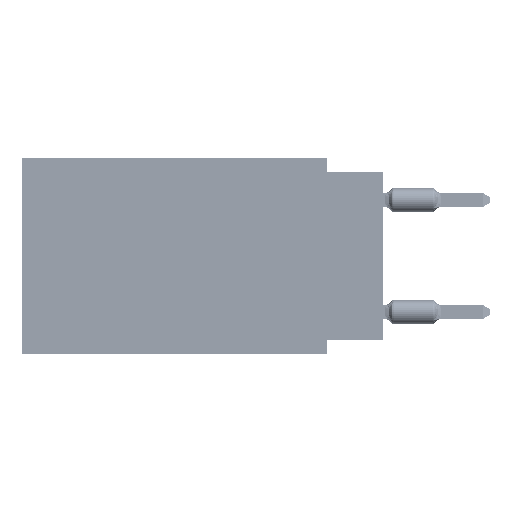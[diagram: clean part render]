
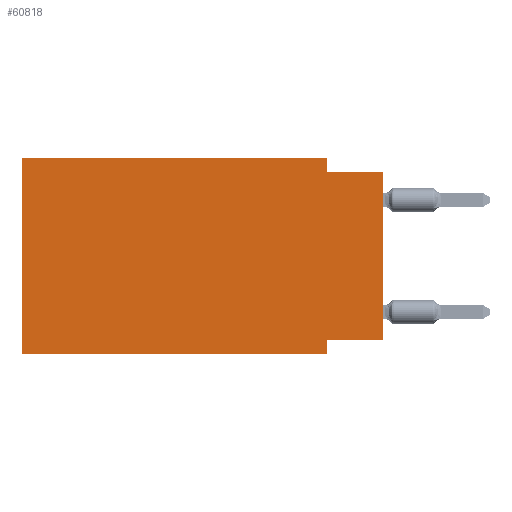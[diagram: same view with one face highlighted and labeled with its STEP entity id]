
A CAD part, left-side view. The second image highlights one B-rep face of the part: STEP entity #60818.
In plain terms, the highlighted planar face has unit normal (-1, 0, 0).
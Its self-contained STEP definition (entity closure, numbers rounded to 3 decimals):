
#2092 = DIRECTION ( 'NONE',  ( 0., -1., 0. ) ) ;
#2361 = LINE ( 'NONE', #91214, #15564 ) ;
#3045 = FACE_OUTER_BOUND ( 'NONE', #11937, .T. ) ;
#4152 = LINE ( 'NONE', #65462, #68832 ) ;
#7784 = CARTESIAN_POINT ( 'NONE',  ( 0., 0., -0.635 ) ) ;
#11937 = EDGE_LOOP ( 'NONE', ( #81461, #65099, #87087, #83864, #63018, #51238, #30250, #26063 ) ) ;
#12713 = AXIS2_PLACEMENT_3D ( 'NONE', #33919, #62898, #18721 ) ;
#15564 = VECTOR ( 'NONE', #53435, 1000. ) ;
#18721 = DIRECTION ( 'NONE',  ( 0., 0., -1. ) ) ;
#24284 = LINE ( 'NONE', #54211, #64107 ) ;
#25144 = CARTESIAN_POINT ( 'NONE',  ( 0., 0., -0.635 ) ) ;
#26063 = ORIENTED_EDGE ( 'NONE', *, *, #83132, .F. ) ;
#26356 = DIRECTION ( 'NONE',  ( 0., 0., 1. ) ) ;
#27761 = EDGE_CURVE ( 'NONE', #49866, #81852, #4152, .T. ) ;
#28850 = VERTEX_POINT ( 'NONE', #36926 ) ;
#29474 = CARTESIAN_POINT ( 'NONE',  ( 0., 2.54, -8.255 ) ) ;
#30038 = VECTOR ( 'NONE', #26356, 1000. ) ;
#30250 = ORIENTED_EDGE ( 'NONE', *, *, #27761, .F. ) ;
#30496 = VECTOR ( 'NONE', #78305, 1000. ) ;
#33228 = LINE ( 'NONE', #71983, #30038 ) ;
#33919 = CARTESIAN_POINT ( 'NONE',  ( 0., 16.383, 0. ) ) ;
#36542 = VERTEX_POINT ( 'NONE', #7784 ) ;
#36926 = CARTESIAN_POINT ( 'NONE',  ( 0., 16.383, 0. ) ) ;
#36971 = EDGE_CURVE ( 'NONE', #58294, #81852, #63474, .T. ) ;
#38929 = VECTOR ( 'NONE', #62022, 1000. ) ;
#42200 = CARTESIAN_POINT ( 'NONE',  ( 0., 16.383, 0. ) ) ;
#42896 = DIRECTION ( 'NONE',  ( 0., 0., -1. ) ) ;
#43327 = VERTEX_POINT ( 'NONE', #69070 ) ;
#44041 = VECTOR ( 'NONE', #2092, 1000. ) ;
#44327 = VERTEX_POINT ( 'NONE', #67769 ) ;
#47376 = LINE ( 'NONE', #62113, #30496 ) ;
#49866 = VERTEX_POINT ( 'NONE', #29474 ) ;
#50780 = EDGE_CURVE ( 'NONE', #59638, #36542, #69331, .T. ) ;
#51238 = ORIENTED_EDGE ( 'NONE', *, *, #36971, .T. ) ;
#51826 = EDGE_CURVE ( 'NONE', #44327, #36542, #33228, .T. ) ;
#53435 = DIRECTION ( 'NONE',  ( 0., 0., -1. ) ) ;
#54211 = CARTESIAN_POINT ( 'NONE',  ( 0., 0., -8.255 ) ) ;
#54282 = VECTOR ( 'NONE', #64767, 1000. ) ;
#58294 = VERTEX_POINT ( 'NONE', #81008 ) ;
#59638 = VERTEX_POINT ( 'NONE', #65173 ) ;
#60818 = ADVANCED_FACE ( 'NONE', ( #3045 ), #63864, .F. ) ;
#62022 = DIRECTION ( 'NONE',  ( 0., -1., 0. ) ) ;
#62113 = CARTESIAN_POINT ( 'NONE',  ( 0., 16.383, 0. ) ) ;
#62898 = DIRECTION ( 'NONE',  ( 1., 0., 0. ) ) ;
#63018 = ORIENTED_EDGE ( 'NONE', *, *, #68877, .F. ) ;
#63474 = LINE ( 'NONE', #86050, #38929 ) ;
#63864 = PLANE ( 'NONE',  #12713 ) ;
#64107 = VECTOR ( 'NONE', #84153, 1000. ) ;
#64767 = DIRECTION ( 'NONE',  ( 0., 0., 1. ) ) ;
#65099 = ORIENTED_EDGE ( 'NONE', *, *, #50780, .F. ) ;
#65148 = EDGE_CURVE ( 'NONE', #28850, #43327, #47376, .T. ) ;
#65173 = CARTESIAN_POINT ( 'NONE',  ( 0., 2.54, -0.635 ) ) ;
#65462 = CARTESIAN_POINT ( 'NONE',  ( 0., 2.54, -8.89 ) ) ;
#67769 = CARTESIAN_POINT ( 'NONE',  ( 0., 0., -8.255 ) ) ;
#68832 = VECTOR ( 'NONE', #42896, 1000. ) ;
#68877 = EDGE_CURVE ( 'NONE', #58294, #28850, #79499, .T. ) ;
#69070 = CARTESIAN_POINT ( 'NONE',  ( 0., 2.54, 0. ) ) ;
#69331 = LINE ( 'NONE', #25144, #44041 ) ;
#71983 = CARTESIAN_POINT ( 'NONE',  ( 0., 0., 0. ) ) ;
#72487 = EDGE_CURVE ( 'NONE', #43327, #59638, #2361, .T. ) ;
#76668 = CARTESIAN_POINT ( 'NONE',  ( 0., 2.54, -8.89 ) ) ;
#78305 = DIRECTION ( 'NONE',  ( 0., -1., 0. ) ) ;
#79499 = LINE ( 'NONE', #42200, #54282 ) ;
#81008 = CARTESIAN_POINT ( 'NONE',  ( 0., 16.383, -8.89 ) ) ;
#81461 = ORIENTED_EDGE ( 'NONE', *, *, #51826, .T. ) ;
#81852 = VERTEX_POINT ( 'NONE', #76668 ) ;
#83132 = EDGE_CURVE ( 'NONE', #44327, #49866, #24284, .T. ) ;
#83864 = ORIENTED_EDGE ( 'NONE', *, *, #65148, .F. ) ;
#84153 = DIRECTION ( 'NONE',  ( 0., 1., 0. ) ) ;
#86050 = CARTESIAN_POINT ( 'NONE',  ( 0., 16.383, -8.89 ) ) ;
#87087 = ORIENTED_EDGE ( 'NONE', *, *, #72487, .F. ) ;
#91214 = CARTESIAN_POINT ( 'NONE',  ( 0., 2.54, 0. ) ) ;
